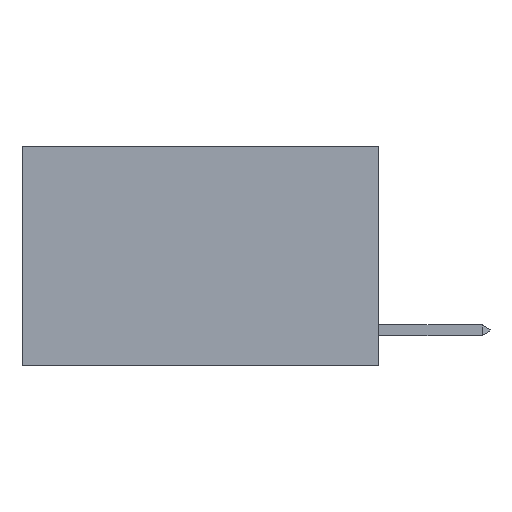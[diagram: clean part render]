
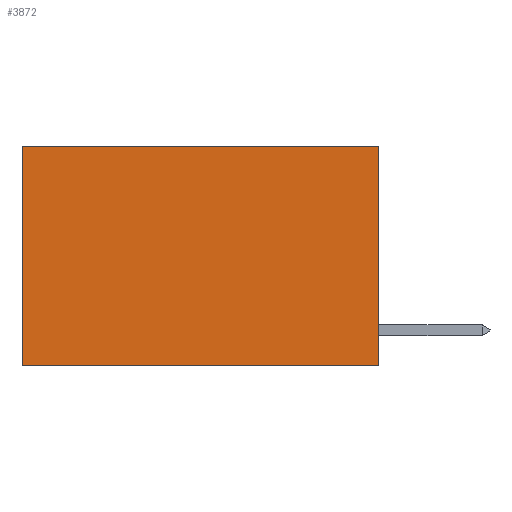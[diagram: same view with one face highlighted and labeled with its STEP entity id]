
A CAD part, left-side view. The second image highlights one B-rep face of the part: STEP entity #3872.
In plain terms, the highlighted planar face has unit normal (-1, 0, 0).
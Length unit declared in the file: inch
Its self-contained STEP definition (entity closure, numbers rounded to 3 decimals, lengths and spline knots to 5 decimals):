
#238 = CARTESIAN_POINT ( 'NONE',  ( 0.2625, 0.6, -0.37 ) ) ;
#974 = EDGE_CURVE ( 'NONE', #14540, #4675, #4319, .T. ) ;
#1886 = VERTEX_POINT ( 'NONE', #9907 ) ;
#2446 = EDGE_CURVE ( 'NONE', #4675, #9663, #15765, .T. ) ;
#3238 = VECTOR ( 'NONE', #11959, 39.37008 ) ;
#3535 = AXIS2_PLACEMENT_3D ( 'NONE', #4366, #4451, #16980 ) ;
#3872 = ADVANCED_FACE ( 'NONE', ( #10958 ), #16284, .F. ) ;
#3967 = DIRECTION ( 'NONE',  ( 0., 0., -1. ) ) ;
#4319 = LINE ( 'NONE', #6696, #3238 ) ;
#4366 = CARTESIAN_POINT ( 'NONE',  ( 0.2625, 0., 0. ) ) ;
#4451 = DIRECTION ( 'NONE',  ( 1., 0., 0. ) ) ;
#4675 = VERTEX_POINT ( 'NONE', #9713 ) ;
#6438 = ORIENTED_EDGE ( 'NONE', *, *, #974, .T. ) ;
#6649 = DIRECTION ( 'NONE',  ( 0., 0., -1. ) ) ;
#6696 = CARTESIAN_POINT ( 'NONE',  ( 0.2625, 0., 0. ) ) ;
#7202 = EDGE_LOOP ( 'NONE', ( #12185, #11101, #15698, #6438 ) ) ;
#7309 = EDGE_CURVE ( 'NONE', #1886, #9663, #11882, .T. ) ;
#7798 = EDGE_CURVE ( 'NONE', #14540, #1886, #17178, .T. ) ;
#8623 = VECTOR ( 'NONE', #15987, 39.37008 ) ;
#9663 = VERTEX_POINT ( 'NONE', #238 ) ;
#9713 = CARTESIAN_POINT ( 'NONE',  ( 0.2625, 0.6, 0. ) ) ;
#9907 = CARTESIAN_POINT ( 'NONE',  ( 0.2625, 0., -0.37 ) ) ;
#10406 = CARTESIAN_POINT ( 'NONE',  ( 0.2625, 0., -0.37 ) ) ;
#10958 = FACE_OUTER_BOUND ( 'NONE', #7202, .T. ) ;
#11101 = ORIENTED_EDGE ( 'NONE', *, *, #7309, .F. ) ;
#11660 = VECTOR ( 'NONE', #3967, 39.37008 ) ;
#11823 = VECTOR ( 'NONE', #6649, 39.37008 ) ;
#11882 = LINE ( 'NONE', #10406, #8623 ) ;
#11959 = DIRECTION ( 'NONE',  ( 0., 1., 0. ) ) ;
#12185 = ORIENTED_EDGE ( 'NONE', *, *, #2446, .T. ) ;
#13460 = CARTESIAN_POINT ( 'NONE',  ( 0.2625, 0.6, 0. ) ) ;
#14361 = CARTESIAN_POINT ( 'NONE',  ( 0.2625, 0., 0. ) ) ;
#14540 = VERTEX_POINT ( 'NONE', #14361 ) ;
#15698 = ORIENTED_EDGE ( 'NONE', *, *, #7798, .F. ) ;
#15765 = LINE ( 'NONE', #13460, #11823 ) ;
#15873 = CARTESIAN_POINT ( 'NONE',  ( 0.2625, 0., 0. ) ) ;
#15987 = DIRECTION ( 'NONE',  ( 0., 1., 0. ) ) ;
#16284 = PLANE ( 'NONE',  #3535 ) ;
#16980 = DIRECTION ( 'NONE',  ( 0., 0., -1. ) ) ;
#17178 = LINE ( 'NONE', #15873, #11660 ) ;
